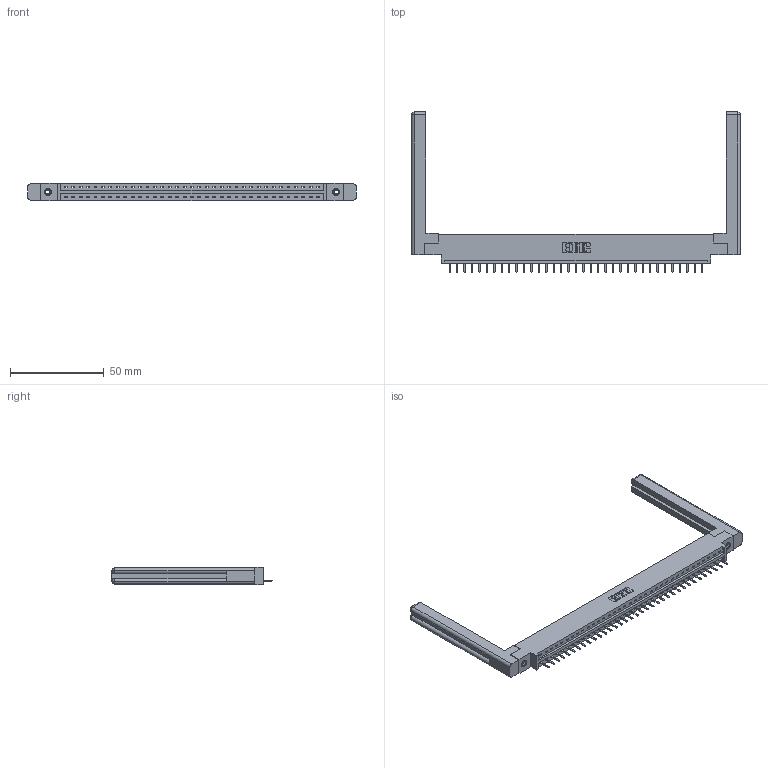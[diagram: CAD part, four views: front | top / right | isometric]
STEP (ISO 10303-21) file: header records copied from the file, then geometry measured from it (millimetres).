
FILE_DESCRIPTION (( 'STEP AP203' ), '1' );
FILE_NAME ('387-035-520-658.STEP', '2019-10-04T11:50:49', ( '' ), ( '' ), 'SwSTEP 2.0', 'SolidWorks 2016', '' );
FILE_SCHEMA (( 'CONFIG_CONTROL_DESIGN' ));
Length unit declared in the file: inch
Products named in the file (5): 345-292-001_345-293-120; 337 Part_0.170 Offset - 0.156 Dia-TI; 387-035-520-658; 307-220-058; 345-250-001_345-250-001-102
Assembly tree (40 placements, depth 2):
  387-035-520-658
    337 Part_0.170 Offset - 0.156 Dia-TI
    345-292-001_345-293-120  x35
    345-250-001_345-250-001-102  x2
    307-220-058  x2
Bounding box: 175.31 x 85.43 x 9.4 mm (x, y, z)
Volume: 25077 mm3; surface area: 23420.5 mm2
Topology: 40 solids, 40 shells, 2570 faces, 7537 edges, 4918 vertices
Faces by surface type: plane 1838, cylinder 708, cone 12, torus 12
Entity records: 29802 total; most frequent: CARTESIAN_POINT 5202, ORIENTED_EDGE 5100, DIRECTION 4400, EDGE_CURVE 2550, VECTOR 2370, LINE 2370, VERTEX_POINT 1690, AXIS2_PLACEMENT_3D 1015
